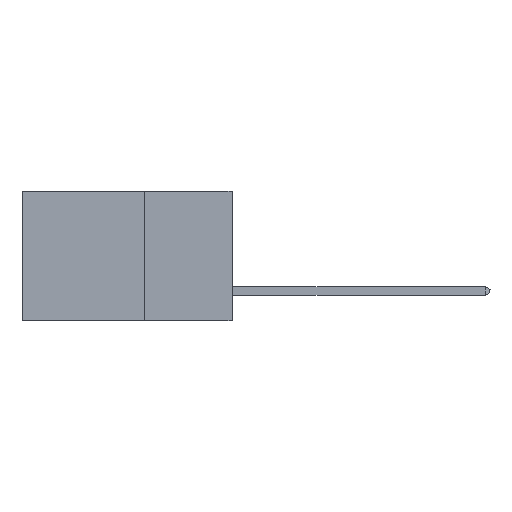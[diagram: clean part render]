
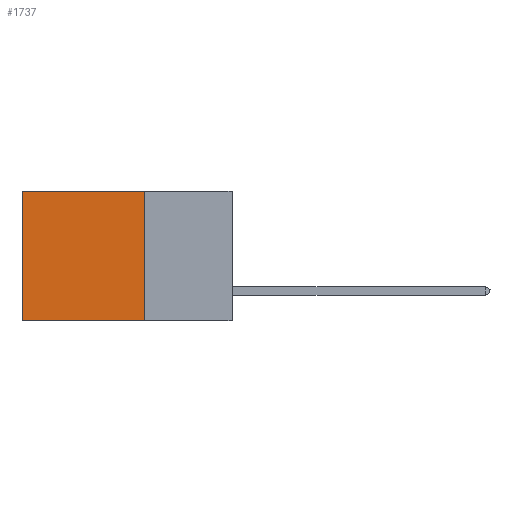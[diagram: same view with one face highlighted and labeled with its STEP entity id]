
A CAD part, left-side view. The second image highlights one B-rep face of the part: STEP entity #1737.
In plain terms, the highlighted planar face has unit normal (-1, 0, 0).
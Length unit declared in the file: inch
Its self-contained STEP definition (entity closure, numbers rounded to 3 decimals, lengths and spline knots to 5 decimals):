
#277 = VECTOR ( 'NONE', #15443, 39.37008 ) ;
#908 = DIRECTION ( 'NONE',  ( 1., 0., 0. ) ) ;
#946 = CARTESIAN_POINT ( 'NONE',  ( 0.2875, 0.25, 0. ) ) ;
#1513 = ORIENTED_EDGE ( 'NONE', *, *, #9362, .F. ) ;
#1565 = ORIENTED_EDGE ( 'NONE', *, *, #2852, .F. ) ;
#1657 = VERTEX_POINT ( 'NONE', #16731 ) ;
#1737 = ADVANCED_FACE ( 'NONE', ( #6525 ), #17928, .F. ) ;
#1754 = AXIS2_PLACEMENT_3D ( 'NONE', #15037, #908, #10752 ) ;
#2330 = ORIENTED_EDGE ( 'NONE', *, *, #9905, .T. ) ;
#2852 = EDGE_CURVE ( 'NONE', #13433, #1657, #8738, .T. ) ;
#4221 = VERTEX_POINT ( 'NONE', #8390 ) ;
#4532 = LINE ( 'NONE', #946, #277 ) ;
#4908 = VECTOR ( 'NONE', #14518, 39.37008 ) ;
#5817 = CARTESIAN_POINT ( 'NONE',  ( 0.2875, 0.25, -0.37 ) ) ;
#6525 = FACE_OUTER_BOUND ( 'NONE', #15065, .T. ) ;
#7407 = CARTESIAN_POINT ( 'NONE',  ( 0.2875, 0.25, 0. ) ) ;
#8281 = VECTOR ( 'NONE', #18180, 39.37008 ) ;
#8390 = CARTESIAN_POINT ( 'NONE',  ( 0.2875, 0.6, 0. ) ) ;
#8738 = LINE ( 'NONE', #12821, #4908 ) ;
#9362 = EDGE_CURVE ( 'NONE', #10806, #13433, #9519, .T. ) ;
#9519 = LINE ( 'NONE', #14306, #15616 ) ;
#9905 = EDGE_CURVE ( 'NONE', #10806, #4221, #4532, .T. ) ;
#10752 = DIRECTION ( 'NONE',  ( 0., 0., -1. ) ) ;
#10806 = VERTEX_POINT ( 'NONE', #7407 ) ;
#11534 = DIRECTION ( 'NONE',  ( 0., 0., -1. ) ) ;
#12562 = EDGE_CURVE ( 'NONE', #4221, #1657, #12807, .T. ) ;
#12807 = LINE ( 'NONE', #18236, #8281 ) ;
#12821 = CARTESIAN_POINT ( 'NONE',  ( 0.2875, 0.25, -0.37 ) ) ;
#13332 = ORIENTED_EDGE ( 'NONE', *, *, #12562, .T. ) ;
#13433 = VERTEX_POINT ( 'NONE', #5817 ) ;
#14306 = CARTESIAN_POINT ( 'NONE',  ( 0.2875, 0.25, 0. ) ) ;
#14518 = DIRECTION ( 'NONE',  ( 0., 1., 0. ) ) ;
#15037 = CARTESIAN_POINT ( 'NONE',  ( 0.2875, 0.25, 0. ) ) ;
#15065 = EDGE_LOOP ( 'NONE', ( #13332, #1565, #1513, #2330 ) ) ;
#15443 = DIRECTION ( 'NONE',  ( 0., 1., 0. ) ) ;
#15616 = VECTOR ( 'NONE', #11534, 39.37008 ) ;
#16731 = CARTESIAN_POINT ( 'NONE',  ( 0.2875, 0.6, -0.37 ) ) ;
#17928 = PLANE ( 'NONE',  #1754 ) ;
#18180 = DIRECTION ( 'NONE',  ( 0., 0., -1. ) ) ;
#18236 = CARTESIAN_POINT ( 'NONE',  ( 0.2875, 0.6, 0. ) ) ;
